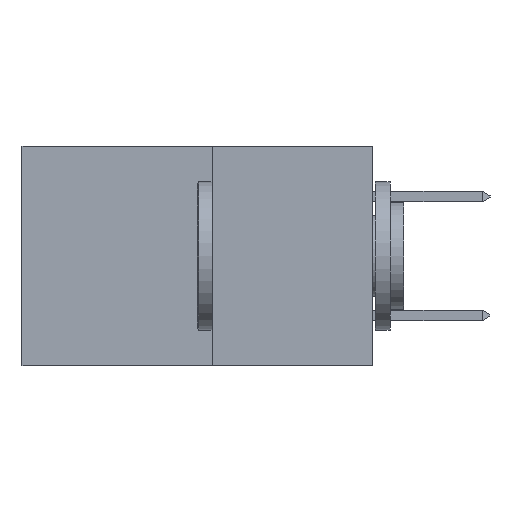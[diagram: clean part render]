
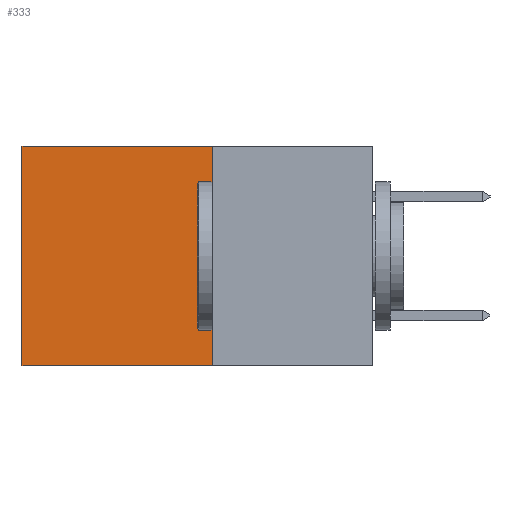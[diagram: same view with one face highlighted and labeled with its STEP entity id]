
A CAD part, left-side view. The second image highlights one B-rep face of the part: STEP entity #333.
In plain terms, the highlighted planar face has unit normal (-1, 0, 0).
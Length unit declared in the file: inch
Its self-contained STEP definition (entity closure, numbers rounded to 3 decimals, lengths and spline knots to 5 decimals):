
#35 = EDGE_CURVE ( 'NONE', #4175, #6896, #5144, .T. ) ;
#333 = ADVANCED_FACE ( 'NONE', ( #3515 ), #2403, .F. ) ;
#423 = ORIENTED_EDGE ( 'NONE', *, *, #8722, .F. ) ;
#1106 = CARTESIAN_POINT ( 'NONE',  ( 0.277, 0.59, -0.37 ) ) ;
#1230 = VECTOR ( 'NONE', #10140, 39.37008 ) ;
#1889 = DIRECTION ( 'NONE',  ( 0., 0., -1. ) ) ;
#2180 = LINE ( 'NONE', #10840, #6392 ) ;
#2403 = PLANE ( 'NONE',  #11556 ) ;
#2637 = ORIENTED_EDGE ( 'NONE', *, *, #35, .T. ) ;
#2899 = ORIENTED_EDGE ( 'NONE', *, *, #10864, .F. ) ;
#2935 = DIRECTION ( 'NONE',  ( 0., 0., -1. ) ) ;
#3515 = FACE_OUTER_BOUND ( 'NONE', #7628, .T. ) ;
#3679 = EDGE_CURVE ( 'NONE', #4821, #4175, #6016, .T. ) ;
#4118 = CARTESIAN_POINT ( 'NONE',  ( 0.277, 0.59, 0. ) ) ;
#4175 = VERTEX_POINT ( 'NONE', #4118 ) ;
#4249 = CARTESIAN_POINT ( 'NONE',  ( 0.277, 0.27, 0. ) ) ;
#4342 = DIRECTION ( 'NONE',  ( 0., 1., 0. ) ) ;
#4422 = CARTESIAN_POINT ( 'NONE',  ( 0.277, 0.27, -0.37 ) ) ;
#4821 = VERTEX_POINT ( 'NONE', #4249 ) ;
#5144 = LINE ( 'NONE', #1106, #9482 ) ;
#5249 = ORIENTED_EDGE ( 'NONE', *, *, #3679, .T. ) ;
#5613 = CARTESIAN_POINT ( 'NONE',  ( 0.277, 0.27, -0.37 ) ) ;
#5705 = DIRECTION ( 'NONE',  ( 1., 0., 0. ) ) ;
#6016 = LINE ( 'NONE', #10334, #1230 ) ;
#6392 = VECTOR ( 'NONE', #1889, 39.37008 ) ;
#6555 = VECTOR ( 'NONE', #4342, 39.37008 ) ;
#6896 = VERTEX_POINT ( 'NONE', #11405 ) ;
#7628 = EDGE_LOOP ( 'NONE', ( #2637, #423, #2899, #5249 ) ) ;
#7840 = VERTEX_POINT ( 'NONE', #5613 ) ;
#8391 = CARTESIAN_POINT ( 'NONE',  ( 0.277, 0.27, -0.37 ) ) ;
#8722 = EDGE_CURVE ( 'NONE', #7840, #6896, #8993, .T. ) ;
#8993 = LINE ( 'NONE', #4422, #6555 ) ;
#9482 = VECTOR ( 'NONE', #2935, 39.37008 ) ;
#10140 = DIRECTION ( 'NONE',  ( 0., 1., 0. ) ) ;
#10334 = CARTESIAN_POINT ( 'NONE',  ( 0.277, 0.27, 0. ) ) ;
#10840 = CARTESIAN_POINT ( 'NONE',  ( 0.277, 0.27, -0.37 ) ) ;
#10864 = EDGE_CURVE ( 'NONE', #4821, #7840, #2180, .T. ) ;
#11031 = DIRECTION ( 'NONE',  ( 0., 0., -1. ) ) ;
#11405 = CARTESIAN_POINT ( 'NONE',  ( 0.277, 0.59, -0.37 ) ) ;
#11556 = AXIS2_PLACEMENT_3D ( 'NONE', #8391, #5705, #11031 ) ;
